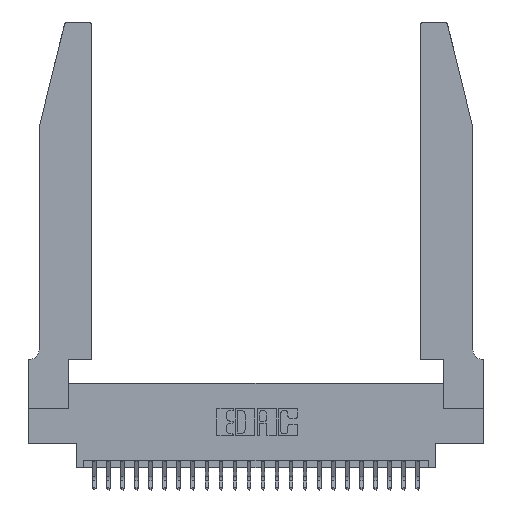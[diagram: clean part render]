
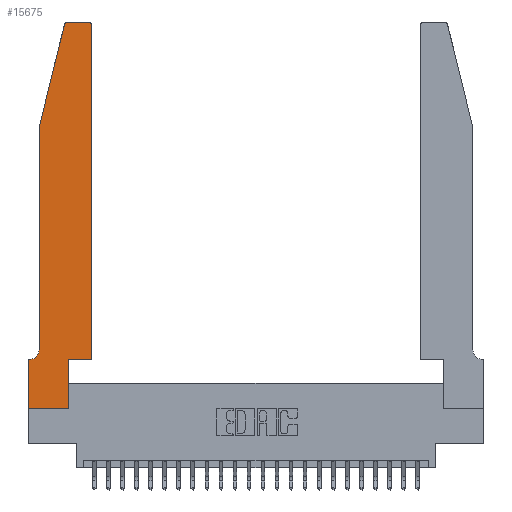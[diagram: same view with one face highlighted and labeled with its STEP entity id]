
A CAD part, top view. The second image highlights one B-rep face of the part: STEP entity #15675.
In plain terms, the highlighted planar face has unit normal (0, 0, 1).
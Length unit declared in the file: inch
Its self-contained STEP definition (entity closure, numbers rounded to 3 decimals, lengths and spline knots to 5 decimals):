
#34 = CARTESIAN_POINT ( 'NONE',  ( 0.4505, 0.35, 0.37 ) ) ;
#459 = CARTESIAN_POINT ( 'NONE',  ( 0.4505, 0.35, 0.37 ) ) ;
#1060 = VERTEX_POINT ( 'NONE', #3530 ) ;
#1294 = CARTESIAN_POINT ( 'NONE',  ( 0.0755, 2., 0.37 ) ) ;
#1301 = DIRECTION ( 'NONE',  ( 0., 1., 0. ) ) ;
#1423 = VECTOR ( 'NONE', #10709, 39.37008 ) ;
#1581 = EDGE_CURVE ( 'NONE', #3668, #12773, #7754, .T. ) ;
#1682 = CARTESIAN_POINT ( 'NONE',  ( 0.4205, 2.72, 0.37 ) ) ;
#1901 = ORIENTED_EDGE ( 'NONE', *, *, #4163, .T. ) ;
#2103 = VECTOR ( 'NONE', #9814, 39.37008 ) ;
#2390 = VECTOR ( 'NONE', #1301, 39.37008 ) ;
#2646 = DIRECTION ( 'NONE',  ( 1., 0., 0. ) ) ;
#2921 = EDGE_CURVE ( 'NONE', #25513, #11882, #17789, .T. ) ;
#3161 = VERTEX_POINT ( 'NONE', #13376 ) ;
#3303 = ORIENTED_EDGE ( 'NONE', *, *, #7611, .T. ) ;
#3513 = CARTESIAN_POINT ( 'NONE',  ( 0.4505, 2.72, 0.37 ) ) ;
#3530 = CARTESIAN_POINT ( 'NONE',  ( 0.0755, 2., 0.37 ) ) ;
#3657 = CIRCLE ( 'NONE', #6400, 0.07 ) ;
#3668 = VERTEX_POINT ( 'NONE', #10365 ) ;
#3880 = DIRECTION ( 'NONE',  ( 1., 0., 0. ) ) ;
#3942 = AXIS2_PLACEMENT_3D ( 'NONE', #18273, #6219, #20252 ) ;
#3984 = CARTESIAN_POINT ( 'NONE',  ( 0.2865, 0., 0.37 ) ) ;
#3985 = ORIENTED_EDGE ( 'NONE', *, *, #1581, .T. ) ;
#4163 = EDGE_CURVE ( 'NONE', #16688, #24464, #12717, .T. ) ;
#4371 = CARTESIAN_POINT ( 'NONE',  ( 0., 0., 0.37 ) ) ;
#5788 = LINE ( 'NONE', #7541, #10580 ) ;
#5790 = EDGE_CURVE ( 'NONE', #6546, #3161, #19342, .T. ) ;
#5798 = VERTEX_POINT ( 'NONE', #8197 ) ;
#5924 = DIRECTION ( 'NONE',  ( 0., 0., 1. ) ) ;
#5961 = DIRECTION ( 'NONE',  ( -1., 0., 0. ) ) ;
#5982 = ORIENTED_EDGE ( 'NONE', *, *, #6185, .T. ) ;
#6185 = EDGE_CURVE ( 'NONE', #11882, #3668, #5788, .T. ) ;
#6219 = DIRECTION ( 'NONE',  ( 0., 0., 1. ) ) ;
#6298 = DIRECTION ( 'NONE',  ( 0., -1., 0. ) ) ;
#6384 = FACE_OUTER_BOUND ( 'NONE', #20713, .T. ) ;
#6400 = AXIS2_PLACEMENT_3D ( 'NONE', #21976, #10050, #23987 ) ;
#6546 = VERTEX_POINT ( 'NONE', #14629 ) ;
#7541 = CARTESIAN_POINT ( 'NONE',  ( 0.2865, 0.35, 0.37 ) ) ;
#7591 = CARTESIAN_POINT ( 'NONE',  ( 0.0055, 0.35, 0.37 ) ) ;
#7611 = EDGE_CURVE ( 'NONE', #24464, #25513, #22351, .T. ) ;
#7665 = DIRECTION ( 'NONE',  ( -1., 0., 0. ) ) ;
#7725 = DIRECTION ( 'NONE',  ( -0.239, -0.971, 0. ) ) ;
#7754 = LINE ( 'NONE', #34, #22443 ) ;
#8197 = CARTESIAN_POINT ( 'NONE',  ( 0.0755, 0.42, 0.37 ) ) ;
#9194 = EDGE_CURVE ( 'NONE', #5798, #16688, #3657, .T. ) ;
#9814 = DIRECTION ( 'NONE',  ( 0., -1., 0. ) ) ;
#10025 = LINE ( 'NONE', #1294, #25287 ) ;
#10050 = DIRECTION ( 'NONE',  ( 0., 0., -1. ) ) ;
#10365 = CARTESIAN_POINT ( 'NONE',  ( 0.2865, 0.35, 0.37 ) ) ;
#10580 = VECTOR ( 'NONE', #19554, 39.37008 ) ;
#10709 = DIRECTION ( 'NONE',  ( 1., 0., 0. ) ) ;
#10746 = CARTESIAN_POINT ( 'NONE',  ( 0., 0., 0.37 ) ) ;
#11882 = VERTEX_POINT ( 'NONE', #3984 ) ;
#11995 = PLANE ( 'NONE',  #25462 ) ;
#12381 = CARTESIAN_POINT ( 'NONE',  ( 0.4205, 2.75, 0.37 ) ) ;
#12717 = LINE ( 'NONE', #19752, #22669 ) ;
#12773 = VERTEX_POINT ( 'NONE', #459 ) ;
#13376 = CARTESIAN_POINT ( 'NONE',  ( 0.25487, 2.72718, 0.37 ) ) ;
#13682 = VERTEX_POINT ( 'NONE', #3513 ) ;
#14629 = CARTESIAN_POINT ( 'NONE',  ( 0.284, 2.75, 0.37 ) ) ;
#14814 = ORIENTED_EDGE ( 'NONE', *, *, #2921, .T. ) ;
#15072 = ORIENTED_EDGE ( 'NONE', *, *, #9194, .T. ) ;
#15675 = ADVANCED_FACE ( 'NONE', ( #6384 ), #11995, .T. ) ;
#16060 = DIRECTION ( 'NONE',  ( 0., 0., 1. ) ) ;
#16356 = VERTEX_POINT ( 'NONE', #12381 ) ;
#16532 = AXIS2_PLACEMENT_3D ( 'NONE', #1682, #16060, #3880 ) ;
#16688 = VERTEX_POINT ( 'NONE', #7591 ) ;
#17085 = VECTOR ( 'NONE', #6298, 39.37008 ) ;
#17789 = LINE ( 'NONE', #10746, #1423 ) ;
#17892 = ORIENTED_EDGE ( 'NONE', *, *, #21421, .T. ) ;
#17994 = CARTESIAN_POINT ( 'NONE',  ( 0., 0.35, 0.37 ) ) ;
#18273 = CARTESIAN_POINT ( 'NONE',  ( 0.284, 2.72, 0.37 ) ) ;
#18290 = VECTOR ( 'NONE', #5961, 39.37008 ) ;
#18436 = EDGE_CURVE ( 'NONE', #3161, #1060, #10025, .T. ) ;
#18908 = LINE ( 'NONE', #22015, #18290 ) ;
#19082 = EDGE_CURVE ( 'NONE', #13682, #16356, #26173, .T. ) ;
#19129 = ORIENTED_EDGE ( 'NONE', *, *, #18436, .T. ) ;
#19342 = CIRCLE ( 'NONE', #3942, 0.03 ) ;
#19554 = DIRECTION ( 'NONE',  ( 0., 1., 0. ) ) ;
#19637 = EDGE_CURVE ( 'NONE', #1060, #5798, #23043, .T. ) ;
#19752 = CARTESIAN_POINT ( 'NONE',  ( 0.0755, 0.35, 0.37 ) ) ;
#19754 = ORIENTED_EDGE ( 'NONE', *, *, #19637, .T. ) ;
#19904 = LINE ( 'NONE', #25633, #2390 ) ;
#19971 = DIRECTION ( 'NONE',  ( 1., 0., 0. ) ) ;
#20252 = DIRECTION ( 'NONE',  ( 1., 0., 0. ) ) ;
#20307 = EDGE_CURVE ( 'NONE', #12773, #13682, #19904, .T. ) ;
#20685 = ORIENTED_EDGE ( 'NONE', *, *, #20307, .T. ) ;
#20713 = EDGE_LOOP ( 'NONE', ( #17892, #23157, #19129, #19754, #15072, #1901, #3303, #14814, #5982, #3985, #20685, #25696 ) ) ;
#21247 = CARTESIAN_POINT ( 'NONE',  ( 0., 0.35, 0.37 ) ) ;
#21421 = EDGE_CURVE ( 'NONE', #16356, #6546, #18908, .T. ) ;
#21754 = CARTESIAN_POINT ( 'NONE',  ( 0.0755, 2., 0.37 ) ) ;
#21976 = CARTESIAN_POINT ( 'NONE',  ( 0.0055, 0.42, 0.37 ) ) ;
#22015 = CARTESIAN_POINT ( 'NONE',  ( 0.2605, 2.75, 0.37 ) ) ;
#22248 = CARTESIAN_POINT ( 'NONE',  ( 0., 0., 0.37 ) ) ;
#22351 = LINE ( 'NONE', #22248, #17085 ) ;
#22443 = VECTOR ( 'NONE', #2646, 39.37008 ) ;
#22669 = VECTOR ( 'NONE', #7665, 39.37008 ) ;
#23043 = LINE ( 'NONE', #21754, #2103 ) ;
#23157 = ORIENTED_EDGE ( 'NONE', *, *, #5790, .T. ) ;
#23987 = DIRECTION ( 'NONE',  ( -1., 0., 0. ) ) ;
#24464 = VERTEX_POINT ( 'NONE', #21247 ) ;
#25287 = VECTOR ( 'NONE', #7725, 39.37008 ) ;
#25462 = AXIS2_PLACEMENT_3D ( 'NONE', #17994, #5924, #19971 ) ;
#25513 = VERTEX_POINT ( 'NONE', #4371 ) ;
#25633 = CARTESIAN_POINT ( 'NONE',  ( 0.4505, 0.35, 0.37 ) ) ;
#25696 = ORIENTED_EDGE ( 'NONE', *, *, #19082, .T. ) ;
#26173 = CIRCLE ( 'NONE', #16532, 0.03 ) ;
